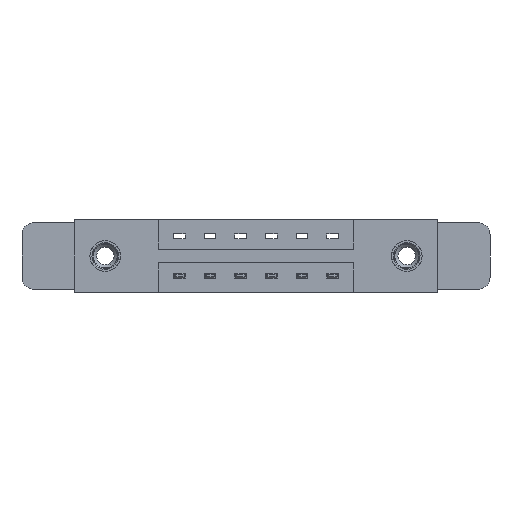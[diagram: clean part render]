
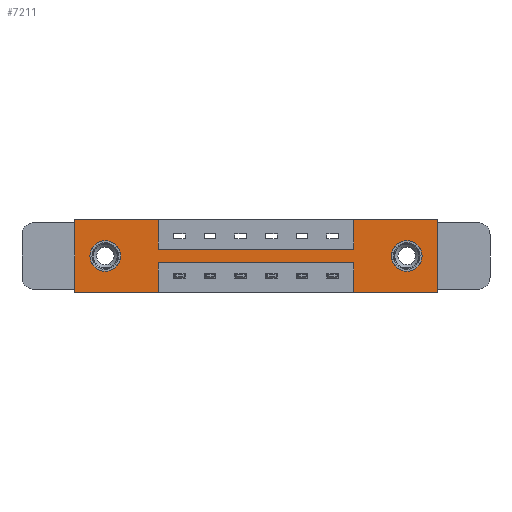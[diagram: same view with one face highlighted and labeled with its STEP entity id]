
A CAD part, front view. The second image highlights one B-rep face of the part: STEP entity #7211.
In plain terms, the highlighted planar face has unit normal (0, -1, 0).
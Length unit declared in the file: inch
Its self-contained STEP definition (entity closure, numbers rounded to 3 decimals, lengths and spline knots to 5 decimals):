
#110 = AXIS2_PLACEMENT_3D ( 'NONE', #6573, #283, #1187 ) ;
#211 = ORIENTED_EDGE ( 'NONE', *, *, #560, .F. ) ;
#225 = VECTOR ( 'NONE', #3648, 39.37008 ) ;
#266 = VERTEX_POINT ( 'NONE', #10914 ) ;
#279 = EDGE_CURVE ( 'NONE', #2107, #10815, #10122, .T. ) ;
#283 = DIRECTION ( 'NONE',  ( 0., -1., 0. ) ) ;
#293 = CARTESIAN_POINT ( 'NONE',  ( 0., 0., -0.37 ) ) ;
#316 = CARTESIAN_POINT ( 'NONE',  ( 1.417, 0., -0.22 ) ) ;
#484 = DIRECTION ( 'NONE',  ( 0., 0., 1. ) ) ;
#560 = EDGE_CURVE ( 'NONE', #2936, #5539, #4937, .T. ) ;
#725 = VECTOR ( 'NONE', #8182, 39.37008 ) ;
#865 = EDGE_CURVE ( 'NONE', #7736, #7848, #6197, .T. ) ;
#1074 = EDGE_CURVE ( 'NONE', #5539, #8341, #7858, .T. ) ;
#1104 = DIRECTION ( 'NONE',  ( 0., 1., 0. ) ) ;
#1187 = DIRECTION ( 'NONE',  ( 0., 0., -1. ) ) ;
#1274 = CARTESIAN_POINT ( 'NONE',  ( 0.155, 0., -0.185 ) ) ;
#1347 = EDGE_CURVE ( 'NONE', #4753, #2936, #11354, .T. ) ;
#1369 = VECTOR ( 'NONE', #484, 39.37008 ) ;
#1502 = DIRECTION ( 'NONE',  ( -1., 0., 0. ) ) ;
#1578 = CARTESIAN_POINT ( 'NONE',  ( 1.687, 0., -0.107 ) ) ;
#1690 = CARTESIAN_POINT ( 'NONE',  ( 0.425, 0., -0.22 ) ) ;
#1763 = EDGE_CURVE ( 'NONE', #5197, #8019, #8289, .T. ) ;
#1949 = DIRECTION ( 'NONE',  ( 0., 1., 0. ) ) ;
#2012 = CARTESIAN_POINT ( 'NONE',  ( 0.155, 0., -0.263 ) ) ;
#2061 = VECTOR ( 'NONE', #6007, 39.37008 ) ;
#2107 = VERTEX_POINT ( 'NONE', #2012 ) ;
#2109 = DIRECTION ( 'NONE',  ( 0., 1., 0. ) ) ;
#2214 = AXIS2_PLACEMENT_3D ( 'NONE', #9780, #1104, #4717 ) ;
#2238 = CARTESIAN_POINT ( 'NONE',  ( 0.425, 0., -0.15 ) ) ;
#2272 = DIRECTION ( 'NONE',  ( 0., 1., 0. ) ) ;
#2286 = VECTOR ( 'NONE', #11452, 39.37008 ) ;
#2318 = DIRECTION ( 'NONE',  ( 0., 0., -1. ) ) ;
#2624 = LINE ( 'NONE', #4693, #225 ) ;
#2683 = CARTESIAN_POINT ( 'NONE',  ( 1.842, 0., 0. ) ) ;
#2809 = LINE ( 'NONE', #5990, #9610 ) ;
#2823 = ORIENTED_EDGE ( 'NONE', *, *, #3723, .F. ) ;
#2877 = VECTOR ( 'NONE', #5464, 39.37008 ) ;
#2886 = VECTOR ( 'NONE', #10736, 39.37008 ) ;
#2936 = VERTEX_POINT ( 'NONE', #10820 ) ;
#2941 = DIRECTION ( 'NONE',  ( 0., 0., -1. ) ) ;
#3042 = CIRCLE ( 'NONE', #5478, 0.078 ) ;
#3434 = CARTESIAN_POINT ( 'NONE',  ( 1.417, 0., -0.37 ) ) ;
#3501 = EDGE_CURVE ( 'NONE', #10815, #2107, #11019, .T. ) ;
#3648 = DIRECTION ( 'NONE',  ( 0., 0., -1. ) ) ;
#3723 = EDGE_CURVE ( 'NONE', #4042, #4753, #2809, .T. ) ;
#4042 = VERTEX_POINT ( 'NONE', #316 ) ;
#4069 = ORIENTED_EDGE ( 'NONE', *, *, #865, .F. ) ;
#4266 = ORIENTED_EDGE ( 'NONE', *, *, #7561, .F. ) ;
#4407 = ORIENTED_EDGE ( 'NONE', *, *, #279, .T. ) ;
#4499 = AXIS2_PLACEMENT_3D ( 'NONE', #7321, #1949, #10845 ) ;
#4591 = VERTEX_POINT ( 'NONE', #5814 ) ;
#4682 = EDGE_CURVE ( 'NONE', #6189, #4042, #6779, .T. ) ;
#4693 = CARTESIAN_POINT ( 'NONE',  ( 0.425, 0., 0. ) ) ;
#4717 = DIRECTION ( 'NONE',  ( 0., 0., 1. ) ) ;
#4753 = VERTEX_POINT ( 'NONE', #1690 ) ;
#4786 = CARTESIAN_POINT ( 'NONE',  ( 1.842, 0., 0. ) ) ;
#4937 = LINE ( 'NONE', #10537, #2286 ) ;
#4973 = VERTEX_POINT ( 'NONE', #2683 ) ;
#5044 = EDGE_CURVE ( 'NONE', #11431, #7736, #2624, .T. ) ;
#5071 = FACE_BOUND ( 'NONE', #7501, .T. ) ;
#5197 = VERTEX_POINT ( 'NONE', #1578 ) ;
#5209 = CARTESIAN_POINT ( 'NONE',  ( 0.425, 0., -0.15 ) ) ;
#5231 = EDGE_LOOP ( 'NONE', ( #9559, #2823, #7772, #4266, #10289, #6239, #9970, #4069, #11085, #9373, #9873, #211 ) ) ;
#5251 = CARTESIAN_POINT ( 'NONE',  ( 1.417, 0., -0.15 ) ) ;
#5258 = EDGE_CURVE ( 'NONE', #8019, #5197, #3042, .T. ) ;
#5320 = CARTESIAN_POINT ( 'NONE',  ( 0., 0., -0.37 ) ) ;
#5464 = DIRECTION ( 'NONE',  ( 0., 0., 1. ) ) ;
#5478 = AXIS2_PLACEMENT_3D ( 'NONE', #9457, #2272, #2318 ) ;
#5539 = VERTEX_POINT ( 'NONE', #5320 ) ;
#5762 = VECTOR ( 'NONE', #7618, 39.37008 ) ;
#5814 = CARTESIAN_POINT ( 'NONE',  ( 1.417, 0., 0. ) ) ;
#5830 = DIRECTION ( 'NONE',  ( 0., 0., 1. ) ) ;
#5990 = CARTESIAN_POINT ( 'NONE',  ( 0.425, 0., -0.22 ) ) ;
#6007 = DIRECTION ( 'NONE',  ( 0., 0., 1. ) ) ;
#6044 = CARTESIAN_POINT ( 'NONE',  ( 0.155, 0., -0.107 ) ) ;
#6189 = VERTEX_POINT ( 'NONE', #9740 ) ;
#6197 = LINE ( 'NONE', #2238, #5762 ) ;
#6239 = ORIENTED_EDGE ( 'NONE', *, *, #9748, .F. ) ;
#6326 = LINE ( 'NONE', #293, #9522 ) ;
#6425 = CARTESIAN_POINT ( 'NONE',  ( 0.425, 0., -0.37 ) ) ;
#6573 = CARTESIAN_POINT ( 'NONE',  ( 0., 0., -0.37 ) ) ;
#6578 = VECTOR ( 'NONE', #2941, 39.37008 ) ;
#6666 = LINE ( 'NONE', #7422, #8624 ) ;
#6779 = LINE ( 'NONE', #3434, #2061 ) ;
#6913 = ORIENTED_EDGE ( 'NONE', *, *, #1763, .T. ) ;
#6978 = EDGE_CURVE ( 'NONE', #8341, #11431, #10245, .T. ) ;
#6980 = LINE ( 'NONE', #4786, #6578 ) ;
#7211 = ADVANCED_FACE ( 'NONE', ( #5071, #10506, #7309 ), #8340, .T. ) ;
#7309 = FACE_OUTER_BOUND ( 'NONE', #5231, .T. ) ;
#7321 = CARTESIAN_POINT ( 'NONE',  ( 1.687, 0., -0.185 ) ) ;
#7422 = CARTESIAN_POINT ( 'NONE',  ( 0., 0., 0. ) ) ;
#7501 = EDGE_LOOP ( 'NONE', ( #6913, #8745 ) ) ;
#7561 = EDGE_CURVE ( 'NONE', #266, #6189, #6326, .T. ) ;
#7618 = DIRECTION ( 'NONE',  ( 1., 0., 0. ) ) ;
#7736 = VERTEX_POINT ( 'NONE', #5209 ) ;
#7772 = ORIENTED_EDGE ( 'NONE', *, *, #4682, .F. ) ;
#7848 = VERTEX_POINT ( 'NONE', #5251 ) ;
#7858 = LINE ( 'NONE', #9943, #2877 ) ;
#8019 = VERTEX_POINT ( 'NONE', #9770 ) ;
#8182 = DIRECTION ( 'NONE',  ( 0., 0., -1. ) ) ;
#8241 = CARTESIAN_POINT ( 'NONE',  ( 0.425, 0., 0. ) ) ;
#8289 = CIRCLE ( 'NONE', #4499, 0.078 ) ;
#8340 = PLANE ( 'NONE',  #110 ) ;
#8341 = VERTEX_POINT ( 'NONE', #9660 ) ;
#8359 = DIRECTION ( 'NONE',  ( 1., 0., 0. ) ) ;
#8372 = AXIS2_PLACEMENT_3D ( 'NONE', #1274, #2109, #5830 ) ;
#8555 = EDGE_CURVE ( 'NONE', #4973, #266, #6980, .T. ) ;
#8624 = VECTOR ( 'NONE', #8359, 39.37008 ) ;
#8671 = CARTESIAN_POINT ( 'NONE',  ( 1.417, 0., 0. ) ) ;
#8745 = ORIENTED_EDGE ( 'NONE', *, *, #5258, .T. ) ;
#9272 = EDGE_CURVE ( 'NONE', #7848, #4591, #9351, .T. ) ;
#9351 = LINE ( 'NONE', #8671, #1369 ) ;
#9373 = ORIENTED_EDGE ( 'NONE', *, *, #6978, .F. ) ;
#9457 = CARTESIAN_POINT ( 'NONE',  ( 1.687, 0., -0.185 ) ) ;
#9522 = VECTOR ( 'NONE', #11077, 39.37008 ) ;
#9559 = ORIENTED_EDGE ( 'NONE', *, *, #1347, .F. ) ;
#9610 = VECTOR ( 'NONE', #1502, 39.37008 ) ;
#9660 = CARTESIAN_POINT ( 'NONE',  ( 0., 0., 0. ) ) ;
#9740 = CARTESIAN_POINT ( 'NONE',  ( 1.417, 0., -0.37 ) ) ;
#9748 = EDGE_CURVE ( 'NONE', #4591, #4973, #6666, .T. ) ;
#9770 = CARTESIAN_POINT ( 'NONE',  ( 1.687, 0., -0.263 ) ) ;
#9780 = CARTESIAN_POINT ( 'NONE',  ( 0.155, 0., -0.185 ) ) ;
#9873 = ORIENTED_EDGE ( 'NONE', *, *, #1074, .F. ) ;
#9943 = CARTESIAN_POINT ( 'NONE',  ( 0., 0., 0. ) ) ;
#9970 = ORIENTED_EDGE ( 'NONE', *, *, #9272, .F. ) ;
#10122 = CIRCLE ( 'NONE', #2214, 0.078 ) ;
#10245 = LINE ( 'NONE', #10697, #2886 ) ;
#10289 = ORIENTED_EDGE ( 'NONE', *, *, #8555, .F. ) ;
#10506 = FACE_BOUND ( 'NONE', #10826, .T. ) ;
#10537 = CARTESIAN_POINT ( 'NONE',  ( 0., 0., -0.37 ) ) ;
#10697 = CARTESIAN_POINT ( 'NONE',  ( 0., 0., 0. ) ) ;
#10736 = DIRECTION ( 'NONE',  ( 1., 0., 0. ) ) ;
#10815 = VERTEX_POINT ( 'NONE', #6044 ) ;
#10820 = CARTESIAN_POINT ( 'NONE',  ( 0.425, 0., -0.37 ) ) ;
#10826 = EDGE_LOOP ( 'NONE', ( #11551, #4407 ) ) ;
#10845 = DIRECTION ( 'NONE',  ( 0., 0., -1. ) ) ;
#10914 = CARTESIAN_POINT ( 'NONE',  ( 1.842, 0., -0.37 ) ) ;
#11019 = CIRCLE ( 'NONE', #8372, 0.078 ) ;
#11077 = DIRECTION ( 'NONE',  ( -1., 0., 0. ) ) ;
#11085 = ORIENTED_EDGE ( 'NONE', *, *, #5044, .F. ) ;
#11354 = LINE ( 'NONE', #6425, #725 ) ;
#11431 = VERTEX_POINT ( 'NONE', #8241 ) ;
#11452 = DIRECTION ( 'NONE',  ( -1., 0., 0. ) ) ;
#11551 = ORIENTED_EDGE ( 'NONE', *, *, #3501, .T. ) ;
